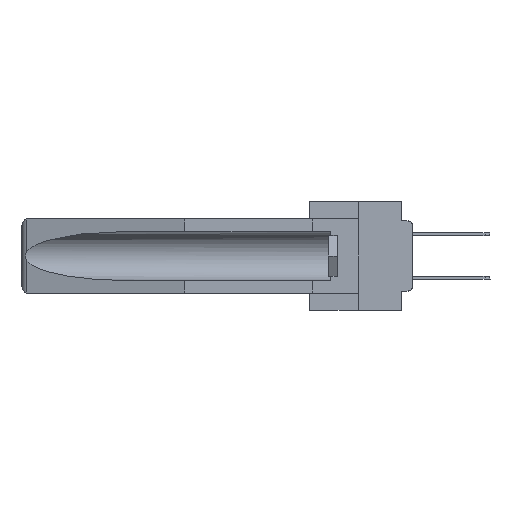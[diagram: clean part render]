
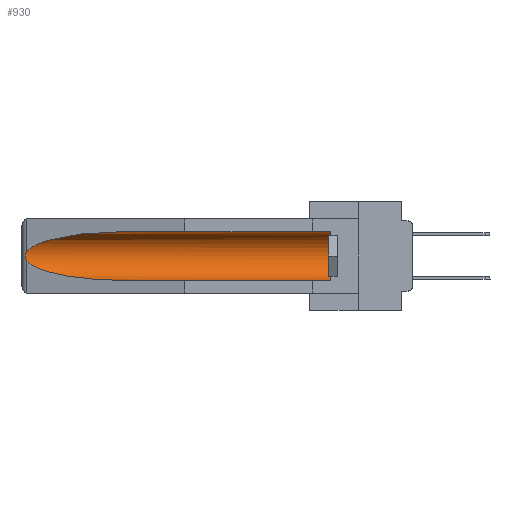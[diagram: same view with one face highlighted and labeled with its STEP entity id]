
A CAD part, left-side view. The second image highlights one B-rep face of the part: STEP entity #930.
In plain terms, the highlighted cylindrical face has radius 2.857 mm (diameter 5.715 mm), a partial arc.
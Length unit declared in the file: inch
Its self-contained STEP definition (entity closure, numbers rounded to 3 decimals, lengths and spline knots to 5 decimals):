
#194 = CARTESIAN_POINT ( 'NONE',  ( 0.25451, 1.48313, -0.09465 ) ) ;
#581 = DIRECTION ( 'NONE',  ( 0., 0., 1. ) ) ;
#930 = ADVANCED_FACE ( 'NONE', ( #4824 ), #19875, .F. ) ;
#1469 = VERTEX_POINT ( 'NONE', #34737 ) ;
#2285 = VERTEX_POINT ( 'NONE', #16677 ) ;
#2663 = CIRCLE ( 'NONE', #18305, 0.1125 ) ;
#3773 = VERTEX_POINT ( 'NONE', #13310 ) ;
#4824 = FACE_OUTER_BOUND ( 'NONE', #23974, .T. ) ;
#4857 = DIRECTION ( 'NONE',  ( 0., 1., 0. ) ) ;
#5302 = VECTOR ( 'NONE', #22434, 39.37008 ) ;
#5636 = VERTEX_POINT ( 'NONE', #16524 ) ;
#7477 =( BOUNDED_CURVE ( )  B_SPLINE_CURVE ( 3, ( #13523, #33295, #35899, #10751 ),
 .UNSPECIFIED., .F., .F. ) 
 B_SPLINE_CURVE_WITH_KNOTS ( ( 4, 4 ),
 ( 0.1948, 1.5708 ),
 .UNSPECIFIED. ) 
 CURVE ( )  GEOMETRIC_REPRESENTATION_ITEM ( )  RATIONAL_B_SPLINE_CURVE ( ( 1., 0.848, 0.848, 1. ) ) 
 REPRESENTATION_ITEM ( '' )  );
#7852 = CARTESIAN_POINT ( 'NONE',  ( 0.155, -0.30754, -0.1715 ) ) ;
#8615 = AXIS2_PLACEMENT_3D ( 'NONE', #7852, #4857, #24676 ) ;
#9033 = CARTESIAN_POINT ( 'NONE',  ( 0.26597, 1.52961, -0.15275 ) ) ;
#9038 = CARTESIAN_POINT ( 'NONE',  ( 0.155, 0.126, -0.1715 ) ) ;
#9168 = CARTESIAN_POINT ( 'NONE',  ( 0.26597, 1.5296, -0.19026 ) ) ;
#10751 = CARTESIAN_POINT ( 'NONE',  ( 0.155, 1.07973, -0.284 ) ) ;
#10778 = EDGE_CURVE ( 'NONE', #5636, #2285, #2663, .T. ) ;
#11323 = EDGE_CURVE ( 'NONE', #5636, #24020, #13785, .T. ) ;
#11860 = CARTESIAN_POINT ( 'NONE',  ( 0.155, 1.07973, -0.059 ) ) ;
#12153 = CARTESIAN_POINT ( 'NONE',  ( 0.26537, 1.52718, -0.14972 ) ) ;
#12498 = EDGE_CURVE ( 'NONE', #1469, #3773, #34961, .T. ) ;
#12783 = EDGE_CURVE ( 'NONE', #2285, #16637, #18970, .T. ) ;
#13266 = VECTOR ( 'NONE', #33449, 39.37008 ) ;
#13310 = CARTESIAN_POINT ( 'NONE',  ( 0.26537, 1.52718, -0.19328 ) ) ;
#13472 = CARTESIAN_POINT ( 'NONE',  ( 0.155, -0.30754, -0.284 ) ) ;
#13523 = CARTESIAN_POINT ( 'NONE',  ( 0.26537, 1.52718, -0.19328 ) ) ;
#13785 = LINE ( 'NONE', #13472, #5302 ) ;
#14380 = CARTESIAN_POINT ( 'NONE',  ( 0.26537, 1.52718, -0.14972 ) ) ;
#14640 = CARTESIAN_POINT ( 'NONE',  ( 0.2675, 1.53308, -0.17534 ) ) ;
#15118 = ORIENTED_EDGE ( 'NONE', *, *, #16394, .T. ) ;
#15872 = EDGE_CURVE ( 'NONE', #16637, #1469, #26056, .T. ) ;
#16394 = EDGE_CURVE ( 'NONE', #3773, #24020, #7477, .T. ) ;
#16521 = ORIENTED_EDGE ( 'NONE', *, *, #10778, .T. ) ;
#16524 = CARTESIAN_POINT ( 'NONE',  ( 0.155, 0.126, -0.284 ) ) ;
#16637 = VERTEX_POINT ( 'NONE', #11860 ) ;
#16677 = CARTESIAN_POINT ( 'NONE',  ( 0.155, 0.126, -0.059 ) ) ;
#17331 = CARTESIAN_POINT ( 'NONE',  ( 0.155, 1.07973, -0.059 ) ) ;
#17608 = ORIENTED_EDGE ( 'NONE', *, *, #15872, .T. ) ;
#18305 = AXIS2_PLACEMENT_3D ( 'NONE', #9038, #20396, #581 ) ;
#18970 = LINE ( 'NONE', #25370, #13266 ) ;
#19875 = CYLINDRICAL_SURFACE ( 'NONE', #8615, 0.1125 ) ;
#20396 = DIRECTION ( 'NONE',  ( 0., -1., 0. ) ) ;
#20639 = CARTESIAN_POINT ( 'NONE',  ( 0.26537, 1.52718, -0.19328 ) ) ;
#22266 = ORIENTED_EDGE ( 'NONE', *, *, #12498, .T. ) ;
#22434 = DIRECTION ( 'NONE',  ( 0., 1., 0. ) ) ;
#23974 = EDGE_LOOP ( 'NONE', ( #17608, #22266, #15118, #26103, #16521, #36021 ) ) ;
#24020 = VERTEX_POINT ( 'NONE', #24514 ) ;
#24514 = CARTESIAN_POINT ( 'NONE',  ( 0.155, 1.07973, -0.284 ) ) ;
#24676 = DIRECTION ( 'NONE',  ( 0., 0., 1. ) ) ;
#25370 = CARTESIAN_POINT ( 'NONE',  ( 0.155, -0.30754, -0.059 ) ) ;
#25712 = CARTESIAN_POINT ( 'NONE',  ( 0.21114, 1.30732, -0.059 ) ) ;
#25854 = CARTESIAN_POINT ( 'NONE',  ( 0.2675, 1.53308, -0.16763 ) ) ;
#26056 =( BOUNDED_CURVE ( )  B_SPLINE_CURVE ( 3, ( #17331, #25712, #194, #14380 ),
 .UNSPECIFIED., .F., .F. ) 
 B_SPLINE_CURVE_WITH_KNOTS ( ( 4, 4 ),
 ( 4.71239, 6.08839 ),
 .UNSPECIFIED. ) 
 CURVE ( )  GEOMETRIC_REPRESENTATION_ITEM ( )  RATIONAL_B_SPLINE_CURVE ( ( 1., 0.848, 0.848, 1. ) ) 
 REPRESENTATION_ITEM ( '' )  );
#26079 = CARTESIAN_POINT ( 'NONE',  ( 0.2673, 1.5327, -0.16383 ) ) ;
#26103 = ORIENTED_EDGE ( 'NONE', *, *, #11323, .F. ) ;
#28838 = CARTESIAN_POINT ( 'NONE',  ( 0.26655, 1.53094, -0.18657 ) ) ;
#31934 = CARTESIAN_POINT ( 'NONE',  ( 0.26654, 1.53092, -0.15636 ) ) ;
#33295 = CARTESIAN_POINT ( 'NONE',  ( 0.25451, 1.48313, -0.24835 ) ) ;
#33449 = DIRECTION ( 'NONE',  ( 0., 1., 0. ) ) ;
#34737 = CARTESIAN_POINT ( 'NONE',  ( 0.26537, 1.52718, -0.14972 ) ) ;
#34794 = CARTESIAN_POINT ( 'NONE',  ( 0.2673, 1.53269, -0.17917 ) ) ;
#34961 = B_SPLINE_CURVE_WITH_KNOTS ( 'NONE', 3,
 ( #12153, #9033, #31934, #26079, #25854, #14640, #34794, #28838, #9168, #20639 ),
 .UNSPECIFIED., .F., .F.,
 ( 4, 2, 2, 2, 4 ),
 ( 0., 0.00029, 0.00058, 0.00087, 0.00117 ),
 .UNSPECIFIED. ) ;
#35899 = CARTESIAN_POINT ( 'NONE',  ( 0.21114, 1.30732, -0.284 ) ) ;
#36021 = ORIENTED_EDGE ( 'NONE', *, *, #12783, .T. ) ;
